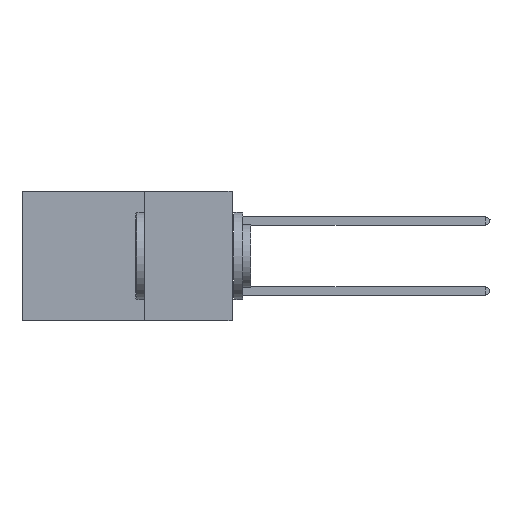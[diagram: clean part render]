
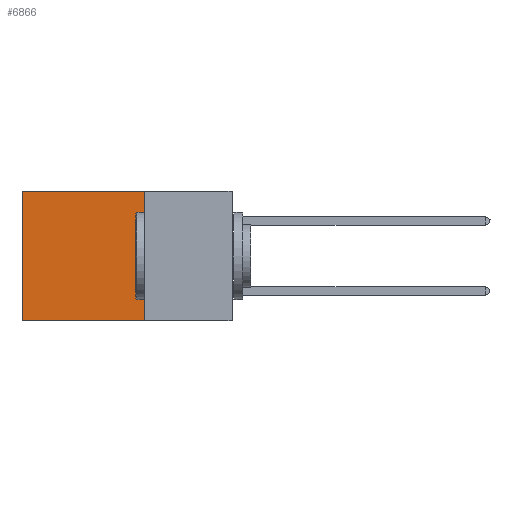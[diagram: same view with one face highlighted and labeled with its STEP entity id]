
A CAD part, left-side view. The second image highlights one B-rep face of the part: STEP entity #6866.
In plain terms, the highlighted planar face has unit normal (-1, 0, 0).
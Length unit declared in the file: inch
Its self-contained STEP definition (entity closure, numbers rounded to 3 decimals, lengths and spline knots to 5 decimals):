
#154 = LINE ( 'NONE', #26239, #10987 ) ;
#512 = CARTESIAN_POINT ( 'NONE',  ( 0.2875, 0.25, -0.37 ) ) ;
#1236 = VECTOR ( 'NONE', #26842, 39.37008 ) ;
#1942 = DIRECTION ( 'NONE',  ( 0., 0., -1. ) ) ;
#2019 = AXIS2_PLACEMENT_3D ( 'NONE', #11366, #19412, #1942 ) ;
#3734 = DIRECTION ( 'NONE',  ( 0., 1., 0. ) ) ;
#3773 = EDGE_CURVE ( 'NONE', #14965, #16117, #14825, .T. ) ;
#6265 = LINE ( 'NONE', #21910, #1236 ) ;
#6866 = ADVANCED_FACE ( 'NONE', ( #13428 ), #13540, .F. ) ;
#8353 = CARTESIAN_POINT ( 'NONE',  ( 0.2875, 0.6, 0. ) ) ;
#8885 = ORIENTED_EDGE ( 'NONE', *, *, #3773, .T. ) ;
#10276 = ORIENTED_EDGE ( 'NONE', *, *, #14373, .T. ) ;
#10987 = VECTOR ( 'NONE', #3734, 39.37008 ) ;
#11018 = LINE ( 'NONE', #24103, #20345 ) ;
#11366 = CARTESIAN_POINT ( 'NONE',  ( 0.2875, 0.25, 0. ) ) ;
#13428 = FACE_OUTER_BOUND ( 'NONE', #26860, .T. ) ;
#13540 = PLANE ( 'NONE',  #2019 ) ;
#14094 = EDGE_CURVE ( 'NONE', #14291, #20640, #11018, .T. ) ;
#14136 = CARTESIAN_POINT ( 'NONE',  ( 0.2875, 0.6, 0. ) ) ;
#14291 = VERTEX_POINT ( 'NONE', #20661 ) ;
#14373 = EDGE_CURVE ( 'NONE', #14291, #14965, #154, .T. ) ;
#14825 = LINE ( 'NONE', #14136, #20282 ) ;
#14965 = VERTEX_POINT ( 'NONE', #8353 ) ;
#15033 = CARTESIAN_POINT ( 'NONE',  ( 0.2875, 0.6, -0.37 ) ) ;
#15367 = EDGE_CURVE ( 'NONE', #20640, #16117, #6265, .T. ) ;
#16117 = VERTEX_POINT ( 'NONE', #15033 ) ;
#19412 = DIRECTION ( 'NONE',  ( 1., 0., 0. ) ) ;
#20282 = VECTOR ( 'NONE', #31408, 39.37008 ) ;
#20345 = VECTOR ( 'NONE', #26517, 39.37008 ) ;
#20640 = VERTEX_POINT ( 'NONE', #512 ) ;
#20661 = CARTESIAN_POINT ( 'NONE',  ( 0.2875, 0.25, 0. ) ) ;
#21910 = CARTESIAN_POINT ( 'NONE',  ( 0.2875, 0.25, -0.37 ) ) ;
#22105 = ORIENTED_EDGE ( 'NONE', *, *, #15367, .F. ) ;
#22263 = ORIENTED_EDGE ( 'NONE', *, *, #14094, .F. ) ;
#24103 = CARTESIAN_POINT ( 'NONE',  ( 0.2875, 0.25, 0. ) ) ;
#26239 = CARTESIAN_POINT ( 'NONE',  ( 0.2875, 0.25, 0. ) ) ;
#26517 = DIRECTION ( 'NONE',  ( 0., 0., -1. ) ) ;
#26842 = DIRECTION ( 'NONE',  ( 0., 1., 0. ) ) ;
#26860 = EDGE_LOOP ( 'NONE', ( #8885, #22105, #22263, #10276 ) ) ;
#31408 = DIRECTION ( 'NONE',  ( 0., 0., -1. ) ) ;
